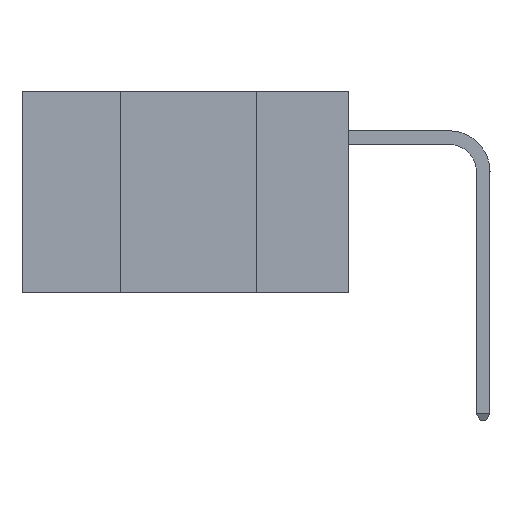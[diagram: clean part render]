
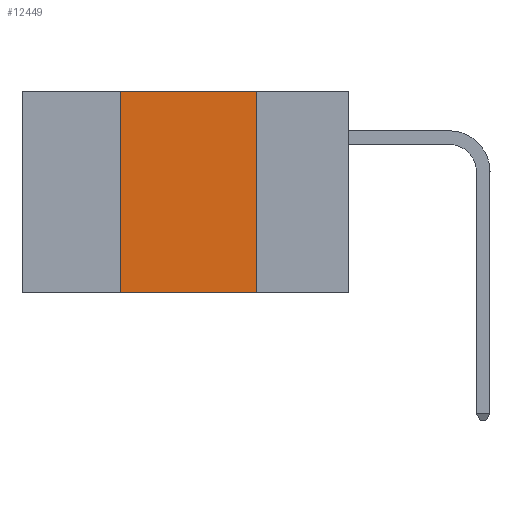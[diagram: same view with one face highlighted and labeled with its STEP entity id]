
A CAD part, left-side view. The second image highlights one B-rep face of the part: STEP entity #12449.
In plain terms, the highlighted planar face has unit normal (-1, 0, 0).
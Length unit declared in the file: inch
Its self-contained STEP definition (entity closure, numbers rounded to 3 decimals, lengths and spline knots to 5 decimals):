
#72 = VERTEX_POINT ( 'NONE', #19873 ) ;
#339 = VERTEX_POINT ( 'NONE', #20907 ) ;
#780 = AXIS2_PLACEMENT_3D ( 'NONE', #28636, #31789, #13045 ) ;
#3390 = CARTESIAN_POINT ( 'NONE',  ( 0., 0.42, 0. ) ) ;
#9354 = VECTOR ( 'NONE', #17031, 39.37008 ) ;
#9487 = DIRECTION ( 'NONE',  ( 0., 0., -1. ) ) ;
#9548 = CARTESIAN_POINT ( 'NONE',  ( 0., 0.6, -0.37 ) ) ;
#10830 = FACE_OUTER_BOUND ( 'NONE', #25672, .T. ) ;
#11867 = VECTOR ( 'NONE', #15293, 39.37008 ) ;
#12449 = ADVANCED_FACE ( 'NONE', ( #10830 ), #19903, .F. ) ;
#13045 = DIRECTION ( 'NONE',  ( 0., 0., -1. ) ) ;
#14352 = CARTESIAN_POINT ( 'NONE',  ( 0., 0.42, -0.37 ) ) ;
#15293 = DIRECTION ( 'NONE',  ( 0., -1., 0. ) ) ;
#16963 = ORIENTED_EDGE ( 'NONE', *, *, #38351, .F. ) ;
#17031 = DIRECTION ( 'NONE',  ( 0., 0., 1. ) ) ;
#17229 = VECTOR ( 'NONE', #37684, 39.37008 ) ;
#17645 = ORIENTED_EDGE ( 'NONE', *, *, #19219, .T. ) ;
#19084 = VERTEX_POINT ( 'NONE', #14352 ) ;
#19219 = EDGE_CURVE ( 'NONE', #19084, #72, #21135, .T. ) ;
#19232 = VERTEX_POINT ( 'NONE', #3390 ) ;
#19574 = VECTOR ( 'NONE', #9487, 39.37008 ) ;
#19772 = CARTESIAN_POINT ( 'NONE',  ( 0., 0.42, 0. ) ) ;
#19873 = CARTESIAN_POINT ( 'NONE',  ( 0., 0.17, -0.37 ) ) ;
#19903 = PLANE ( 'NONE',  #780 ) ;
#20907 = CARTESIAN_POINT ( 'NONE',  ( 0., 0.17, 0. ) ) ;
#21135 = LINE ( 'NONE', #9548, #17229 ) ;
#25185 = ORIENTED_EDGE ( 'NONE', *, *, #32705, .F. ) ;
#25672 = EDGE_LOOP ( 'NONE', ( #38611, #16963, #25185, #17645 ) ) ;
#28012 = CARTESIAN_POINT ( 'NONE',  ( 0., 0.6, 0. ) ) ;
#28636 = CARTESIAN_POINT ( 'NONE',  ( 0., 0.6, 0. ) ) ;
#31789 = DIRECTION ( 'NONE',  ( 1., 0., 0. ) ) ;
#32277 = LINE ( 'NONE', #34635, #19574 ) ;
#32705 = EDGE_CURVE ( 'NONE', #19084, #19232, #32861, .T. ) ;
#32861 = LINE ( 'NONE', #19772, #9354 ) ;
#34635 = CARTESIAN_POINT ( 'NONE',  ( 0., 0.17, 0. ) ) ;
#36257 = LINE ( 'NONE', #28012, #11867 ) ;
#37684 = DIRECTION ( 'NONE',  ( 0., -1., 0. ) ) ;
#38351 = EDGE_CURVE ( 'NONE', #19232, #339, #36257, .T. ) ;
#38611 = ORIENTED_EDGE ( 'NONE', *, *, #40241, .F. ) ;
#40241 = EDGE_CURVE ( 'NONE', #339, #72, #32277, .T. ) ;
